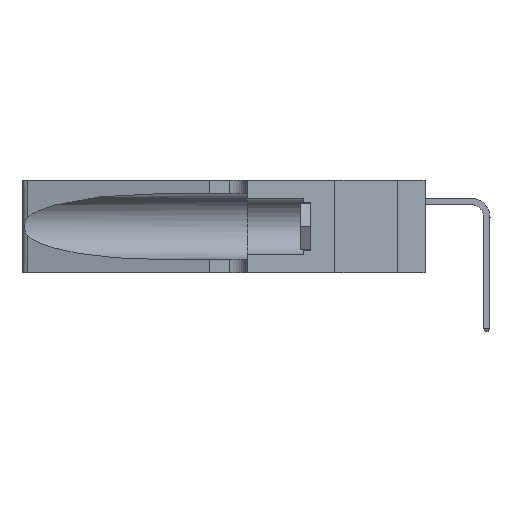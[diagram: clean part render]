
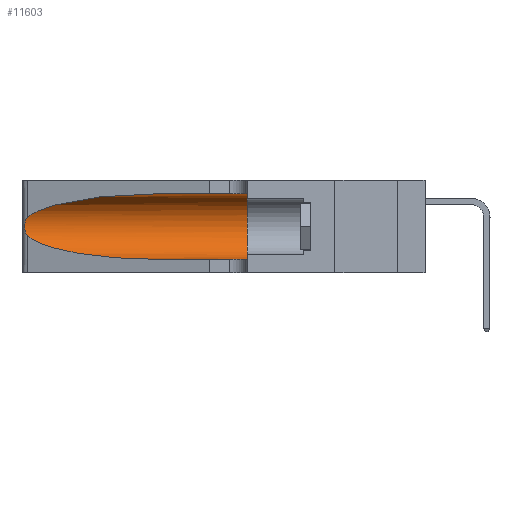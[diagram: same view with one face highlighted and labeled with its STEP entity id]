
A CAD part, left-side view. The second image highlights one B-rep face of the part: STEP entity #11603.
In plain terms, the highlighted cylindrical face has radius 3.308 mm (diameter 6.617 mm), a partial arc.
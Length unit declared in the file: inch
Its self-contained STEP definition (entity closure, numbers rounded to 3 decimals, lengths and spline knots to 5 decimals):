
#36 = ORIENTED_EDGE ( 'NONE', *, *, #4079, .T. ) ;
#138 = CARTESIAN_POINT ( 'NONE',  ( 0.25487, 1.22718, 0.14631 ) ) ;
#148 = CARTESIAN_POINT ( 'NONE',  ( 0.25854, 1.2359, 0.20912 ) ) ;
#221 = CARTESIAN_POINT ( 'NONE',  ( 0.18966, 0.96281, 0.05475 ) ) ;
#1331 = CARTESIAN_POINT ( 'NONE',  ( 0.1305, 0.72297, 0.31525 ) ) ;
#1450 = EDGE_LOOP ( 'NONE', ( #10293, #36, #8610, #12141, #16220, #16868 ) ) ;
#1925 = CARTESIAN_POINT ( 'NONE',  ( 0.26075, 1.23896, 0.19203 ) ) ;
#2100 = AXIS2_PLACEMENT_3D ( 'NONE', #6211, #17395, #7884 ) ;
#2279 = EDGE_CURVE ( 'NONE', #3736, #17396, #10410, .T. ) ;
#3268 = CARTESIAN_POINT ( 'NONE',  ( 0.25487, 1.22718, 0.22369 ) ) ;
#3505 = VECTOR ( 'NONE', #15125, 39.37008 ) ;
#3583 = CARTESIAN_POINT ( 'NONE',  ( 0.26017, 1.23833, 0.17102 ) ) ;
#3629 = CARTESIAN_POINT ( 'NONE',  ( 0.25487, 1.22718, 0.22369 ) ) ;
#3632 = VERTEX_POINT ( 'NONE', #5685 ) ;
#3736 = VERTEX_POINT ( 'NONE', #7640 ) ;
#4079 = EDGE_CURVE ( 'NONE', #15806, #3736, #14089, .T. ) ;
#4630 = CARTESIAN_POINT ( 'NONE',  ( 0.1305, 1.61858, 0.31525 ) ) ;
#5177 = CARTESIAN_POINT ( 'NONE',  ( 0.25487, 1.22718, 0.22369 ) ) ;
#5241 = CARTESIAN_POINT ( 'NONE',  ( 0.25789, 1.23486, 0.15765 ) ) ;
#5685 = CARTESIAN_POINT ( 'NONE',  ( 0.1305, 0.35, 0.31525 ) ) ;
#5746 = VERTEX_POINT ( 'NONE', #1331 ) ;
#6168 = VERTEX_POINT ( 'NONE', #18474 ) ;
#6211 = CARTESIAN_POINT ( 'NONE',  ( 0.1305, 0.35, 0.185 ) ) ;
#6911 = CARTESIAN_POINT ( 'NONE',  ( 0.25555, 1.22993, 0.14849 ) ) ;
#7116 = CARTESIAN_POINT ( 'NONE',  ( 0.1305, 1.61858, 0.05475 ) ) ;
#7144 = EDGE_CURVE ( 'NONE', #5746, #15806, #8226, .T. ) ;
#7532 = EDGE_CURVE ( 'NONE', #3632, #6168, #11025, .T. ) ;
#7640 = CARTESIAN_POINT ( 'NONE',  ( 0.25487, 1.22718, 0.14631 ) ) ;
#7884 = DIRECTION ( 'NONE',  ( 0., 0., 1. ) ) ;
#8163 = CARTESIAN_POINT ( 'NONE',  ( 0.1305, 0.72297, 0.31525 ) ) ;
#8226 =( BOUNDED_CURVE ( )  B_SPLINE_CURVE ( 3, ( #8163, #20887, #12966, #3268 ),
 .UNSPECIFIED., .F., .T. ) 
 B_SPLINE_CURVE_WITH_KNOTS ( ( 4, 4 ),
 ( 1.5708, 2.84003 ),
 .UNSPECIFIED. ) 
 CURVE ( )  GEOMETRIC_REPRESENTATION_ITEM ( )  RATIONAL_B_SPLINE_CURVE ( ( 1., 0.87, 0.87, 1. ) ) 
 REPRESENTATION_ITEM ( '' )  );
#8534 = CARTESIAN_POINT ( 'NONE',  ( 0.2373, 1.15595, 0.08982 ) ) ;
#8588 = CYLINDRICAL_SURFACE ( 'NONE', #9972, 0.13025 ) ;
#8610 = ORIENTED_EDGE ( 'NONE', *, *, #2279, .T. ) ;
#9972 = AXIS2_PLACEMENT_3D ( 'NONE', #20863, #20796, #11348 ) ;
#10085 = CARTESIAN_POINT ( 'NONE',  ( 0.25787, 1.23484, 0.2124 ) ) ;
#10293 = ORIENTED_EDGE ( 'NONE', *, *, #7144, .T. ) ;
#10410 =( BOUNDED_CURVE ( )  B_SPLINE_CURVE ( 3, ( #138, #8534, #221, #11736 ),
 .UNSPECIFIED., .F., .F. ) 
 B_SPLINE_CURVE_WITH_KNOTS ( ( 4, 4 ),
 ( 3.44316, 4.71239 ),
 .UNSPECIFIED. ) 
 CURVE ( )  GEOMETRIC_REPRESENTATION_ITEM ( )  RATIONAL_B_SPLINE_CURVE ( ( 1., 0.87, 0.87, 1. ) ) 
 REPRESENTATION_ITEM ( '' )  );
#10597 = VECTOR ( 'NONE', #12675, 39.37008 ) ;
#11025 = CIRCLE ( 'NONE', #2100, 0.13025 ) ;
#11348 = DIRECTION ( 'NONE',  ( 0., 0., -1. ) ) ;
#11603 = ADVANCED_FACE ( 'NONE', ( #17033 ), #8588, .F. ) ;
#11673 = CARTESIAN_POINT ( 'NONE',  ( 0.26018, 1.23835, 0.19895 ) ) ;
#11736 = CARTESIAN_POINT ( 'NONE',  ( 0.1305, 0.72297, 0.05475 ) ) ;
#12141 = ORIENTED_EDGE ( 'NONE', *, *, #15274, .T. ) ;
#12675 = DIRECTION ( 'NONE',  ( 0., -1., 0. ) ) ;
#12966 = CARTESIAN_POINT ( 'NONE',  ( 0.2373, 1.15595, 0.28018 ) ) ;
#13276 = CARTESIAN_POINT ( 'NONE',  ( 0.26075, 1.23896, 0.178 ) ) ;
#13888 = CARTESIAN_POINT ( 'NONE',  ( 0.1305, 0.72297, 0.05475 ) ) ;
#14089 = B_SPLINE_CURVE_WITH_KNOTS ( 'NONE', 3,
 ( #5177, #14802, #19592, #10085, #148, #11673, #1925, #13276, #3583, #14867, #5241, #16463, #6911, #18060 ),
 .UNSPECIFIED., .F., .F.,
 ( 4, 2, 2, 2, 2, 2, 4 ),
 ( 0., 0.00027, 0.00053, 0.00107, 0.0016, 0.00187, 0.00214 ),
 .UNSPECIFIED. ) ;
#14802 = CARTESIAN_POINT ( 'NONE',  ( 0.25555, 1.22994, 0.2215 ) ) ;
#14867 = CARTESIAN_POINT ( 'NONE',  ( 0.25856, 1.23593, 0.16098 ) ) ;
#15125 = DIRECTION ( 'NONE',  ( 0., -1., 0. ) ) ;
#15274 = EDGE_CURVE ( 'NONE', #17396, #6168, #16354, .T. ) ;
#15306 = LINE ( 'NONE', #4630, #10597 ) ;
#15806 = VERTEX_POINT ( 'NONE', #3629 ) ;
#16194 = EDGE_CURVE ( 'NONE', #5746, #3632, #15306, .T. ) ;
#16220 = ORIENTED_EDGE ( 'NONE', *, *, #7532, .F. ) ;
#16354 = LINE ( 'NONE', #7116, #3505 ) ;
#16463 = CARTESIAN_POINT ( 'NONE',  ( 0.25639, 1.23186, 0.15144 ) ) ;
#16868 = ORIENTED_EDGE ( 'NONE', *, *, #16194, .F. ) ;
#17033 = FACE_OUTER_BOUND ( 'NONE', #1450, .T. ) ;
#17395 = DIRECTION ( 'NONE',  ( 0., 1., 0. ) ) ;
#17396 = VERTEX_POINT ( 'NONE', #13888 ) ;
#18060 = CARTESIAN_POINT ( 'NONE',  ( 0.25487, 1.22718, 0.14631 ) ) ;
#18474 = CARTESIAN_POINT ( 'NONE',  ( 0.1305, 0.35, 0.05475 ) ) ;
#19592 = CARTESIAN_POINT ( 'NONE',  ( 0.25639, 1.23184, 0.21858 ) ) ;
#20796 = DIRECTION ( 'NONE',  ( 0., -1., 0. ) ) ;
#20863 = CARTESIAN_POINT ( 'NONE',  ( 0.1305, 1.61858, 0.185 ) ) ;
#20887 = CARTESIAN_POINT ( 'NONE',  ( 0.18966, 0.96281, 0.31525 ) ) ;
